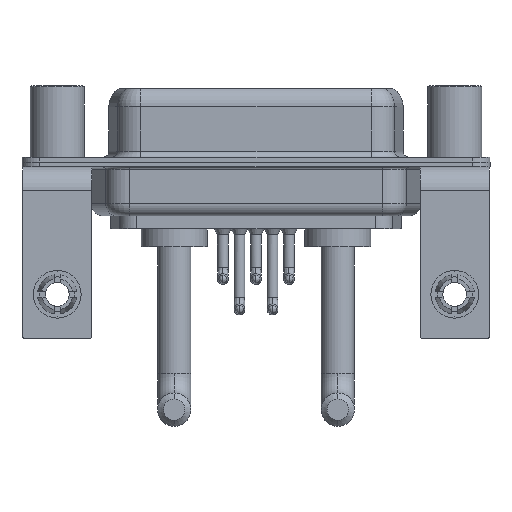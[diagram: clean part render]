
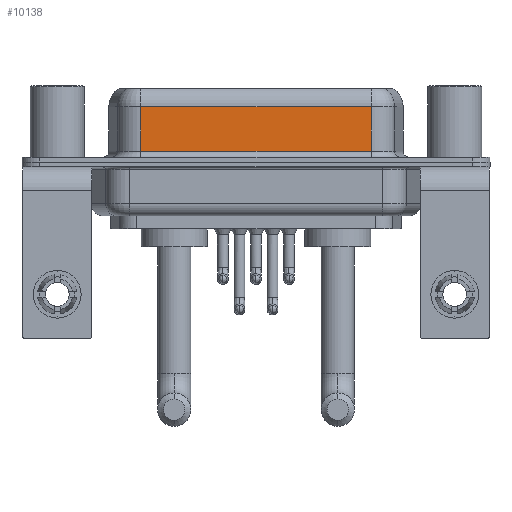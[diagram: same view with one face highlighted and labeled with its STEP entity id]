
A CAD part, front view. The second image highlights one B-rep face of the part: STEP entity #10138.
In plain terms, the highlighted planar face has unit normal (0, -1, 0).
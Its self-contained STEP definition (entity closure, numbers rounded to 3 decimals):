
#260 = CARTESIAN_POINT ( 'NONE',  ( 7.013, -3.95, 6.4 ) ) ;
#1808 = DIRECTION ( 'NONE',  ( 0., 0., 1. ) ) ;
#3059 = CARTESIAN_POINT ( 'NONE',  ( 26.287, -3.95, 6.4 ) ) ;
#4067 = VECTOR ( 'NONE', #5302, 1000. ) ;
#4134 = EDGE_CURVE ( 'NONE', #17912, #10076, #9059, .T. ) ;
#4794 = VERTEX_POINT ( 'NONE', #7143 ) ;
#4895 = LINE ( 'NONE', #260, #19051 ) ;
#5188 = ORIENTED_EDGE ( 'NONE', *, *, #4134, .T. ) ;
#5302 = DIRECTION ( 'NONE',  ( -1., 0., 0. ) ) ;
#5523 = CARTESIAN_POINT ( 'NONE',  ( 7.013, -3.95, 0.9 ) ) ;
#7143 = CARTESIAN_POINT ( 'NONE',  ( 26.287, -3.95, 4.65 ) ) ;
#8314 = DIRECTION ( 'NONE',  ( 0., 0., -1. ) ) ;
#8579 = EDGE_CURVE ( 'NONE', #19994, #17912, #4895, .T. ) ;
#9059 = LINE ( 'NONE', #15466, #18305 ) ;
#9766 = ORIENTED_EDGE ( 'NONE', *, *, #14887, .F. ) ;
#10076 = VERTEX_POINT ( 'NONE', #19083 ) ;
#10138 = ADVANCED_FACE ( 'NONE', ( #17640 ), #11140, .F. ) ;
#11140 = PLANE ( 'NONE',  #14162 ) ;
#11371 = EDGE_LOOP ( 'NONE', ( #9766, #13004, #19273, #5188 ) ) ;
#13004 = ORIENTED_EDGE ( 'NONE', *, *, #14453, .T. ) ;
#13161 = LINE ( 'NONE', #14801, #4067 ) ;
#13242 = LINE ( 'NONE', #19742, #14024 ) ;
#14024 = VECTOR ( 'NONE', #18097, 1000. ) ;
#14162 = AXIS2_PLACEMENT_3D ( 'NONE', #3059, #19180, #1808 ) ;
#14453 = EDGE_CURVE ( 'NONE', #4794, #19994, #13161, .T. ) ;
#14801 = CARTESIAN_POINT ( 'NONE',  ( 26.287, -3.95, 4.65 ) ) ;
#14887 = EDGE_CURVE ( 'NONE', #4794, #10076, #13242, .T. ) ;
#15360 = DIRECTION ( 'NONE',  ( 1., 0., 0. ) ) ;
#15466 = CARTESIAN_POINT ( 'NONE',  ( 26.287, -3.95, 0.9 ) ) ;
#15557 = CARTESIAN_POINT ( 'NONE',  ( 7.013, -3.95, 4.65 ) ) ;
#17640 = FACE_OUTER_BOUND ( 'NONE', #11371, .T. ) ;
#17912 = VERTEX_POINT ( 'NONE', #5523 ) ;
#18097 = DIRECTION ( 'NONE',  ( 0., 0., -1. ) ) ;
#18305 = VECTOR ( 'NONE', #15360, 1000. ) ;
#19051 = VECTOR ( 'NONE', #8314, 1000. ) ;
#19083 = CARTESIAN_POINT ( 'NONE',  ( 26.287, -3.95, 0.9 ) ) ;
#19180 = DIRECTION ( 'NONE',  ( 0., 1., 0. ) ) ;
#19273 = ORIENTED_EDGE ( 'NONE', *, *, #8579, .T. ) ;
#19742 = CARTESIAN_POINT ( 'NONE',  ( 26.287, -3.95, 6.4 ) ) ;
#19994 = VERTEX_POINT ( 'NONE', #15557 ) ;
